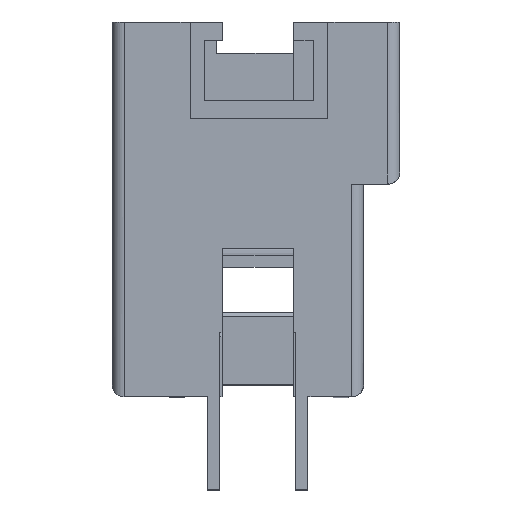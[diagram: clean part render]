
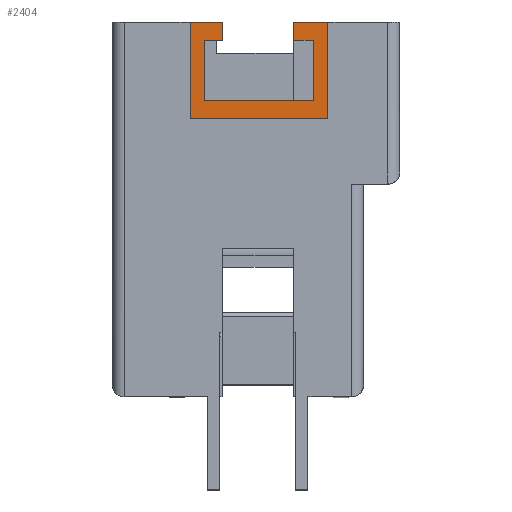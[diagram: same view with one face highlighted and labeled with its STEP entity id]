
A CAD part, top view. The second image highlights one B-rep face of the part: STEP entity #2404.
In plain terms, the highlighted planar face has unit normal (0, 0, 1).
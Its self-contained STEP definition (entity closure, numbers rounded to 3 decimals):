
#58 = DIRECTION ( 'NONE',  ( 1., 0., 0. ) ) ;
#98 = LINE ( 'NONE', #289, #5266 ) ;
#102 = VERTEX_POINT ( 'NONE', #2399 ) ;
#209 = CARTESIAN_POINT ( 'NONE',  ( -11.9, 1.5, 71.2 ) ) ;
#235 = ORIENTED_EDGE ( 'NONE', *, *, #686, .F. ) ;
#251 = CARTESIAN_POINT ( 'NONE',  ( -4.55, -6.234, 71.2 ) ) ;
#270 = LINE ( 'NONE', #3420, #3018 ) ;
#289 = CARTESIAN_POINT ( 'NONE',  ( -13.1, -5., 71.2 ) ) ;
#294 = LINE ( 'NONE', #251, #5458 ) ;
#314 = VECTOR ( 'NONE', #5752, 1000. ) ;
#336 = ORIENTED_EDGE ( 'NONE', *, *, #4995, .T. ) ;
#340 = EDGE_CURVE ( 'NONE', #2418, #2278, #4540, .T. ) ;
#377 = LINE ( 'NONE', #3877, #6519 ) ;
#478 = CARTESIAN_POINT ( 'NONE',  ( -10.45, -6.234, 71.2 ) ) ;
#518 = VERTEX_POINT ( 'NONE', #6559 ) ;
#686 = EDGE_CURVE ( 'NONE', #5600, #5953, #294, .T. ) ;
#750 = DIRECTION ( 'NONE',  ( 0., -1., 0. ) ) ;
#797 = DIRECTION ( 'NONE',  ( 0., 1., 0. ) ) ;
#847 = VECTOR ( 'NONE', #3397, 1000. ) ;
#875 = VERTEX_POINT ( 'NONE', #2643 ) ;
#995 = VECTOR ( 'NONE', #3405, 1000. ) ;
#1046 = DIRECTION ( 'NONE',  ( 0., 0., 1. ) ) ;
#1107 = CARTESIAN_POINT ( 'NONE',  ( -11.9, -3.5, 71.2 ) ) ;
#1110 = CARTESIAN_POINT ( 'NONE',  ( -11.9, -3.5, 71.2 ) ) ;
#1165 = EDGE_CURVE ( 'NONE', #5027, #5793, #6259, .T. ) ;
#1175 = ORIENTED_EDGE ( 'NONE', *, *, #1281, .T. ) ;
#1194 = CARTESIAN_POINT ( 'NONE',  ( -13.1, 3., 71.2 ) ) ;
#1201 = ORIENTED_EDGE ( 'NONE', *, *, #1165, .T. ) ;
#1251 = VECTOR ( 'NONE', #750, 1000. ) ;
#1281 = EDGE_CURVE ( 'NONE', #518, #5027, #270, .T. ) ;
#1409 = EDGE_CURVE ( 'NONE', #3399, #102, #6406, .T. ) ;
#1412 = EDGE_CURVE ( 'NONE', #102, #2418, #2666, .T. ) ;
#1571 = DIRECTION ( 'NONE',  ( 1., 0., 0. ) ) ;
#1586 = EDGE_CURVE ( 'NONE', #875, #4729, #6240, .T. ) ;
#1733 = CARTESIAN_POINT ( 'NONE',  ( -13.1, -5., 71.2 ) ) ;
#1749 = ORIENTED_EDGE ( 'NONE', *, *, #5623, .F. ) ;
#1765 = DIRECTION ( 'NONE',  ( -1., 0., 0. ) ) ;
#1872 = DIRECTION ( 'NONE',  ( -1., 0., 0. ) ) ;
#2129 = ORIENTED_EDGE ( 'NONE', *, *, #6489, .T. ) ;
#2187 = VECTOR ( 'NONE', #5813, 1000. ) ;
#2278 = VERTEX_POINT ( 'NONE', #3064 ) ;
#2399 = CARTESIAN_POINT ( 'NONE',  ( -11.9, 1.5, 71.2 ) ) ;
#2404 = ADVANCED_FACE ( 'NONE', ( #5006 ), #5888, .T. ) ;
#2418 = VERTEX_POINT ( 'NONE', #1107 ) ;
#2457 = ORIENTED_EDGE ( 'NONE', *, *, #4821, .F. ) ;
#2643 = CARTESIAN_POINT ( 'NONE',  ( -1.7, -5., 71.2 ) ) ;
#2655 = CARTESIAN_POINT ( 'NONE',  ( -4.55, 1.5, 71.2 ) ) ;
#2666 = LINE ( 'NONE', #209, #1251 ) ;
#3018 = VECTOR ( 'NONE', #1872, 1000. ) ;
#3064 = CARTESIAN_POINT ( 'NONE',  ( -2.9, -3.5, 71.2 ) ) ;
#3397 = DIRECTION ( 'NONE',  ( 0., -1., 0. ) ) ;
#3399 = VERTEX_POINT ( 'NONE', #5406 ) ;
#3405 = DIRECTION ( 'NONE',  ( 0., 1., 0. ) ) ;
#3420 = CARTESIAN_POINT ( 'NONE',  ( -13.1, 3., 71.2 ) ) ;
#3424 = ORIENTED_EDGE ( 'NONE', *, *, #1409, .F. ) ;
#3463 = ORIENTED_EDGE ( 'NONE', *, *, #1586, .T. ) ;
#3876 = EDGE_CURVE ( 'NONE', #4729, #5953, #4150, .T. ) ;
#3877 = CARTESIAN_POINT ( 'NONE',  ( -11.9, 1.5, 71.2 ) ) ;
#3904 = CARTESIAN_POINT ( 'NONE',  ( -11.9, 1.5, 71.2 ) ) ;
#4103 = VECTOR ( 'NONE', #1765, 1000. ) ;
#4150 = LINE ( 'NONE', #5268, #314 ) ;
#4204 = CARTESIAN_POINT ( 'NONE',  ( -2.9, 1.5, 71.2 ) ) ;
#4230 = CARTESIAN_POINT ( 'NONE',  ( 0., 0., 71.2 ) ) ;
#4257 = CARTESIAN_POINT ( 'NONE',  ( -2.9, 1.5, 71.2 ) ) ;
#4289 = VECTOR ( 'NONE', #58, 1000. ) ;
#4296 = DIRECTION ( 'NONE',  ( 0., 1., 0. ) ) ;
#4454 = CARTESIAN_POINT ( 'NONE',  ( -4.55, 3., 71.2 ) ) ;
#4540 = LINE ( 'NONE', #1110, #4289 ) ;
#4729 = VERTEX_POINT ( 'NONE', #5050 ) ;
#4753 = CARTESIAN_POINT ( 'NONE',  ( -13.1, 3., 71.2 ) ) ;
#4768 = ORIENTED_EDGE ( 'NONE', *, *, #3876, .T. ) ;
#4796 = EDGE_LOOP ( 'NONE', ( #235, #2457, #1749, #5307, #5183, #3424, #336, #1175, #1201, #2129, #3463, #4768 ) ) ;
#4821 = EDGE_CURVE ( 'NONE', #6161, #5600, #377, .T. ) ;
#4995 = EDGE_CURVE ( 'NONE', #3399, #518, #5051, .T. ) ;
#5006 = FACE_OUTER_BOUND ( 'NONE', #4796, .T. ) ;
#5027 = VERTEX_POINT ( 'NONE', #4753 ) ;
#5050 = CARTESIAN_POINT ( 'NONE',  ( -1.7, 3., 71.2 ) ) ;
#5051 = LINE ( 'NONE', #478, #2187 ) ;
#5183 = ORIENTED_EDGE ( 'NONE', *, *, #1412, .F. ) ;
#5266 = VECTOR ( 'NONE', #6139, 1000. ) ;
#5268 = CARTESIAN_POINT ( 'NONE',  ( -13.1, 3., 71.2 ) ) ;
#5307 = ORIENTED_EDGE ( 'NONE', *, *, #340, .F. ) ;
#5406 = CARTESIAN_POINT ( 'NONE',  ( -10.45, 1.5, 71.2 ) ) ;
#5458 = VECTOR ( 'NONE', #797, 1000. ) ;
#5558 = DIRECTION ( 'NONE',  ( -1., 0., 0. ) ) ;
#5600 = VERTEX_POINT ( 'NONE', #2655 ) ;
#5623 = EDGE_CURVE ( 'NONE', #2278, #6161, #5934, .T. ) ;
#5752 = DIRECTION ( 'NONE',  ( -1., 0., 0. ) ) ;
#5793 = VERTEX_POINT ( 'NONE', #1733 ) ;
#5813 = DIRECTION ( 'NONE',  ( 0., 1., 0. ) ) ;
#5888 = PLANE ( 'NONE',  #5980 ) ;
#5934 = LINE ( 'NONE', #4257, #6602 ) ;
#5953 = VERTEX_POINT ( 'NONE', #4454 ) ;
#5980 = AXIS2_PLACEMENT_3D ( 'NONE', #4230, #1046, #1571 ) ;
#6116 = CARTESIAN_POINT ( 'NONE',  ( -1.7, 3., 71.2 ) ) ;
#6139 = DIRECTION ( 'NONE',  ( 1., 0., 0. ) ) ;
#6161 = VERTEX_POINT ( 'NONE', #4204 ) ;
#6240 = LINE ( 'NONE', #6116, #995 ) ;
#6259 = LINE ( 'NONE', #1194, #847 ) ;
#6406 = LINE ( 'NONE', #3904, #4103 ) ;
#6489 = EDGE_CURVE ( 'NONE', #5793, #875, #98, .T. ) ;
#6519 = VECTOR ( 'NONE', #5558, 1000. ) ;
#6559 = CARTESIAN_POINT ( 'NONE',  ( -10.45, 3., 71.2 ) ) ;
#6602 = VECTOR ( 'NONE', #4296, 1000. ) ;
